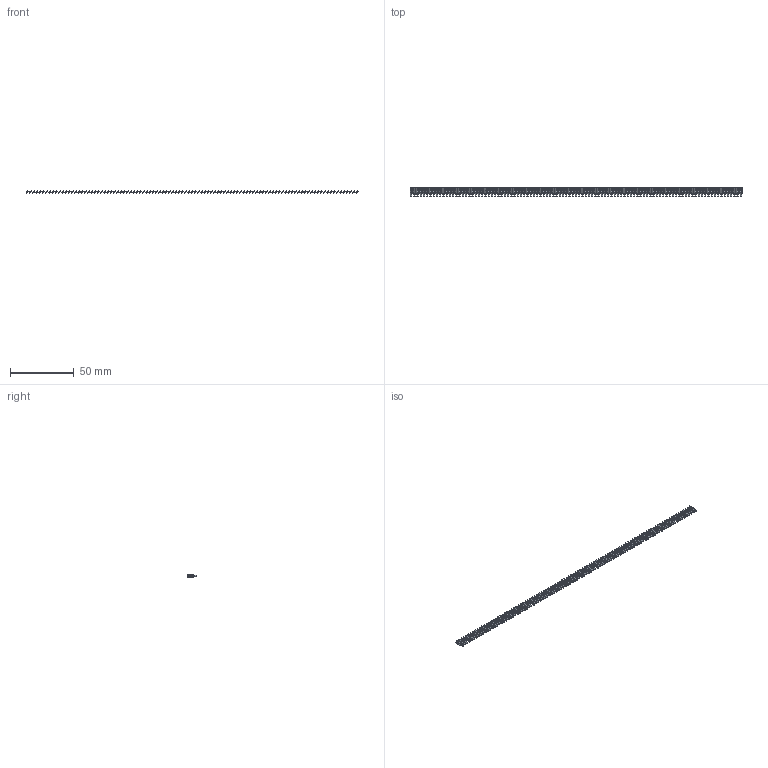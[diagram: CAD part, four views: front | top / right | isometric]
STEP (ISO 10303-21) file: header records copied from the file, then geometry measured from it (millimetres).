
FILE_DESCRIPTION (( 'STEP AP203' ), '1' );
FILE_NAME ('106-103-253-100.STEP', '2020-04-16T23:29:22', ( '' ), ( '' ), 'SwSTEP 2.0', 'SolidWorks 2016', '' );
FILE_SCHEMA (( 'CONFIG_CONTROL_DESIGN' ));
Length unit declared in the file: inch
Products named in the file (2): 100-290-001_100-290-253; 106-103-253-100
Assembly tree (103 placements, depth 2):
  106-103-253-100
    100-290-001_100-290-253  x103
Bounding box: 260.88 x 7.62 x 1.8 mm (x, y, z)
Volume: 568.3 mm3; surface area: 3543.9 mm2
Topology: 103 solids, 103 shells, 2060 faces, 5562 edges, 3708 vertices
Faces by surface type: plane 1957, cylinder 103
Entity records: 4084 total; most frequent: DIRECTION 308, LOCAL_TIME 216, CALENDAR_DATE 216, COORDINATED_UNIVERSAL_TIME_OFFSET 216, CARTESIAN_POINT 216, DATE_AND_TIME 216, AXIS2_PLACEMENT_3D 128, PERSON_AND_ORGANIZATION 119
